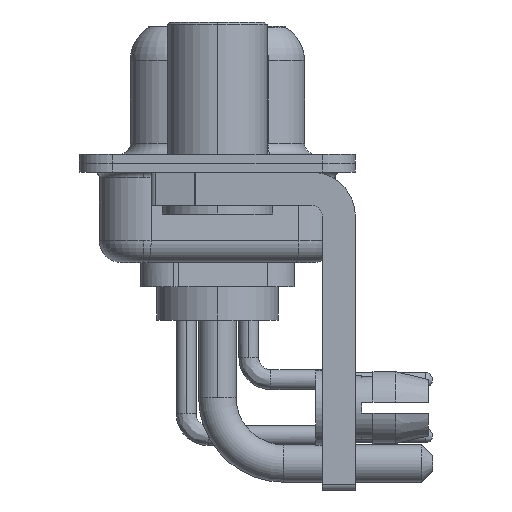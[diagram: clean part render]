
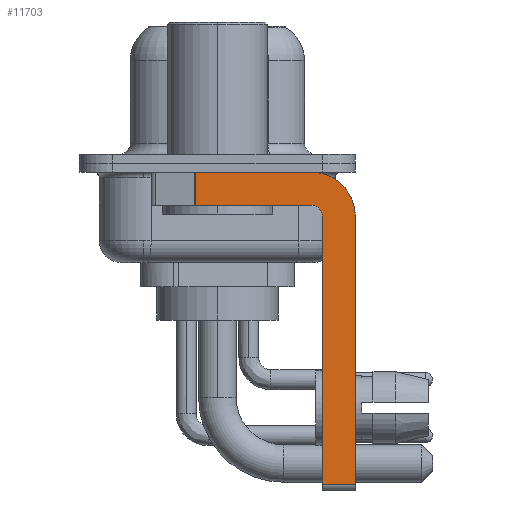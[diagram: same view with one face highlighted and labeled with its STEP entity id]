
A CAD part, left-side view. The second image highlights one B-rep face of the part: STEP entity #11703.
In plain terms, the highlighted planar face has unit normal (-1, 0, 0).
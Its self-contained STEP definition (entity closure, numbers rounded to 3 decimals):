
#13 = VERTEX_POINT ( 'NONE', #9684 ) ;
#88 = CARTESIAN_POINT ( 'NONE',  ( -2.9, 3., -0.4 ) ) ;
#464 = DIRECTION ( 'NONE',  ( 0., 1., 0. ) ) ;
#1452 = DIRECTION ( 'NONE',  ( 0., 0., 1. ) ) ;
#1688 = ORIENTED_EDGE ( 'NONE', *, *, #22363, .F. ) ;
#1717 = LINE ( 'NONE', #18425, #15355 ) ;
#2468 = LINE ( 'NONE', #26764, #7615 ) ;
#3231 = VERTEX_POINT ( 'NONE', #25092 ) ;
#3999 = CARTESIAN_POINT ( 'NONE',  ( -2.9, -4.25, -2.4 ) ) ;
#4324 = VECTOR ( 'NONE', #24570, 1000. ) ;
#4365 = DIRECTION ( 'NONE',  ( 0., 0., -1. ) ) ;
#4469 = LINE ( 'NONE', #17915, #6409 ) ;
#5702 = VERTEX_POINT ( 'NONE', #22141 ) ;
#6409 = VECTOR ( 'NONE', #21727, 1000. ) ;
#6933 = EDGE_CURVE ( 'NONE', #5702, #21968, #4469, .T. ) ;
#7320 = LINE ( 'NONE', #15944, #4324 ) ;
#7493 = ORIENTED_EDGE ( 'NONE', *, *, #9284, .F. ) ;
#7615 = VECTOR ( 'NONE', #18273, 1000. ) ;
#8572 = CARTESIAN_POINT ( 'NONE',  ( -2.9, -4.75, -14.55 ) ) ;
#8609 = CIRCLE ( 'NONE', #25769, 0.5 ) ;
#8863 = DIRECTION ( 'NONE',  ( 0., -1., 0. ) ) ;
#8876 = VERTEX_POINT ( 'NONE', #23826 ) ;
#9096 = EDGE_CURVE ( 'NONE', #22446, #13, #20612, .T. ) ;
#9284 = EDGE_CURVE ( 'NONE', #27183, #22206, #7320, .T. ) ;
#9645 = EDGE_CURVE ( 'NONE', #13, #3231, #2468, .T. ) ;
#9684 = CARTESIAN_POINT ( 'NONE',  ( -2.9, -6.25, -2.4 ) ) ;
#10102 = CARTESIAN_POINT ( 'NONE',  ( -2.9, -4.25, -0.4 ) ) ;
#11127 = AXIS2_PLACEMENT_3D ( 'NONE', #17124, #12626, #21224 ) ;
#11682 = CARTESIAN_POINT ( 'NONE',  ( -2.9, -4.75, -2.4 ) ) ;
#11703 = ADVANCED_FACE ( 'NONE', ( #13009 ), #21908, .F. ) ;
#12307 = ORIENTED_EDGE ( 'NONE', *, *, #6933, .T. ) ;
#12626 = DIRECTION ( 'NONE',  ( 1., 0., 0. ) ) ;
#12829 = EDGE_CURVE ( 'NONE', #8876, #21968, #19856, .T. ) ;
#12846 = LINE ( 'NONE', #88, #17224 ) ;
#13009 = FACE_OUTER_BOUND ( 'NONE', #21209, .T. ) ;
#15125 = DIRECTION ( 'NONE',  ( 1., 0., 0. ) ) ;
#15269 = CARTESIAN_POINT ( 'NONE',  ( -2.9, -4.25, -2.4 ) ) ;
#15355 = VECTOR ( 'NONE', #25337, 1000. ) ;
#15944 = CARTESIAN_POINT ( 'NONE',  ( -2.9, -4.75, -14.8 ) ) ;
#17011 = ORIENTED_EDGE ( 'NONE', *, *, #9096, .F. ) ;
#17124 = CARTESIAN_POINT ( 'NONE',  ( -2.9, -4.25, -2.4 ) ) ;
#17224 = VECTOR ( 'NONE', #8863, 1000. ) ;
#17429 = AXIS2_PLACEMENT_3D ( 'NONE', #15269, #15125, #4365 ) ;
#17915 = CARTESIAN_POINT ( 'NONE',  ( -2.9, 0.978, -1.9 ) ) ;
#18035 = EDGE_CURVE ( 'NONE', #27183, #3231, #1717, .T. ) ;
#18273 = DIRECTION ( 'NONE',  ( 0., 0., -1. ) ) ;
#18425 = CARTESIAN_POINT ( 'NONE',  ( -2.9, -4.25, -14.55 ) ) ;
#19856 = LINE ( 'NONE', #24238, #22842 ) ;
#20612 = CIRCLE ( 'NONE', #11127, 2. ) ;
#20986 = DIRECTION ( 'NONE',  ( -1., 0., 0. ) ) ;
#21209 = EDGE_LOOP ( 'NONE', ( #22623, #12307, #25082, #1688, #7493, #27098, #22343, #17011 ) ) ;
#21224 = DIRECTION ( 'NONE',  ( 0., 0., -1. ) ) ;
#21727 = DIRECTION ( 'NONE',  ( 0., 0., -1. ) ) ;
#21908 = PLANE ( 'NONE',  #17429 ) ;
#21968 = VERTEX_POINT ( 'NONE', #24980 ) ;
#22141 = CARTESIAN_POINT ( 'NONE',  ( -2.9, 0.978, -0.4 ) ) ;
#22206 = VERTEX_POINT ( 'NONE', #11682 ) ;
#22343 = ORIENTED_EDGE ( 'NONE', *, *, #9645, .F. ) ;
#22363 = EDGE_CURVE ( 'NONE', #22206, #8876, #8609, .T. ) ;
#22446 = VERTEX_POINT ( 'NONE', #10102 ) ;
#22623 = ORIENTED_EDGE ( 'NONE', *, *, #23319, .F. ) ;
#22842 = VECTOR ( 'NONE', #464, 1000. ) ;
#23319 = EDGE_CURVE ( 'NONE', #5702, #22446, #12846, .T. ) ;
#23826 = CARTESIAN_POINT ( 'NONE',  ( -2.9, -4.25, -1.9 ) ) ;
#24238 = CARTESIAN_POINT ( 'NONE',  ( -2.9, -4.25, -1.9 ) ) ;
#24570 = DIRECTION ( 'NONE',  ( 0., 0., 1. ) ) ;
#24980 = CARTESIAN_POINT ( 'NONE',  ( -2.9, 0.978, -1.9 ) ) ;
#25082 = ORIENTED_EDGE ( 'NONE', *, *, #12829, .F. ) ;
#25092 = CARTESIAN_POINT ( 'NONE',  ( -2.9, -6.25, -14.55 ) ) ;
#25337 = DIRECTION ( 'NONE',  ( 0., -1., 0. ) ) ;
#25769 = AXIS2_PLACEMENT_3D ( 'NONE', #3999, #20986, #1452 ) ;
#26764 = CARTESIAN_POINT ( 'NONE',  ( -2.9, -6.25, -2.4 ) ) ;
#27098 = ORIENTED_EDGE ( 'NONE', *, *, #18035, .T. ) ;
#27183 = VERTEX_POINT ( 'NONE', #8572 ) ;
